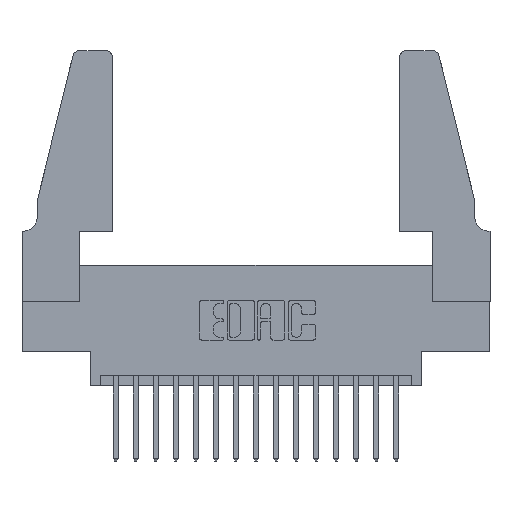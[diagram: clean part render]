
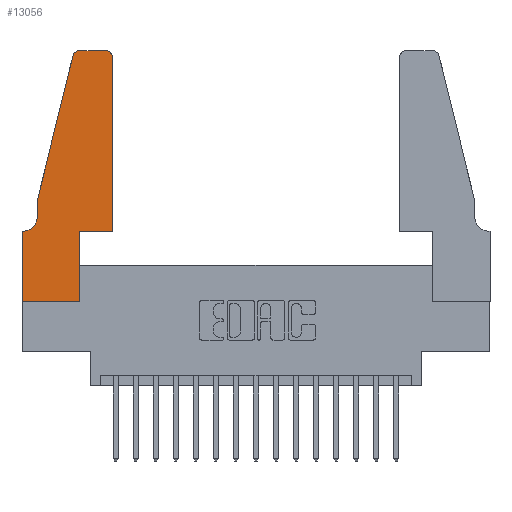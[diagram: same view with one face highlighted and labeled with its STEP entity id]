
A CAD part, top view. The second image highlights one B-rep face of the part: STEP entity #13056.
In plain terms, the highlighted planar face has unit normal (0, 0, 1).
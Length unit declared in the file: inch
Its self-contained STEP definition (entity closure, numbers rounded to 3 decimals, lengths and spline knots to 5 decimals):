
#598 = CARTESIAN_POINT ( 'NONE',  ( 0., 0., 0.37 ) ) ;
#627 = DIRECTION ( 'NONE',  ( -1., 0., 0. ) ) ;
#652 = DIRECTION ( 'NONE',  ( 0., 0., -1. ) ) ;
#676 = CARTESIAN_POINT ( 'NONE',  ( 0.0055, 0.42, 0.37 ) ) ;
#725 = VECTOR ( 'NONE', #9759, 39.37008 ) ;
#914 = VERTEX_POINT ( 'NONE', #3808 ) ;
#1017 = CARTESIAN_POINT ( 'NONE',  ( 0.2605, 1.25, 0.37 ) ) ;
#1130 = LINE ( 'NONE', #12833, #12560 ) ;
#1386 = ORIENTED_EDGE ( 'NONE', *, *, #15940, .T. ) ;
#1443 = EDGE_CURVE ( 'NONE', #9566, #13053, #5546, .T. ) ;
#1550 = ORIENTED_EDGE ( 'NONE', *, *, #2956, .T. ) ;
#1926 = ORIENTED_EDGE ( 'NONE', *, *, #15184, .T. ) ;
#1958 = VERTEX_POINT ( 'NONE', #2604 ) ;
#2333 = CARTESIAN_POINT ( 'NONE',  ( 0.0755, 0.42, 0.37 ) ) ;
#2424 = VERTEX_POINT ( 'NONE', #8724 ) ;
#2604 = CARTESIAN_POINT ( 'NONE',  ( 0.0755, 0.5, 0.37 ) ) ;
#2956 = EDGE_CURVE ( 'NONE', #2424, #6470, #9075, .T. ) ;
#3036 = CIRCLE ( 'NONE', #10200, 0.03 ) ;
#3119 = LINE ( 'NONE', #12220, #16553 ) ;
#3122 = ORIENTED_EDGE ( 'NONE', *, *, #3976, .T. ) ;
#3142 = VERTEX_POINT ( 'NONE', #12787 ) ;
#3474 = VECTOR ( 'NONE', #9433, 39.37008 ) ;
#3808 = CARTESIAN_POINT ( 'NONE',  ( 0.4505, 0.35, 0.37 ) ) ;
#3949 = DIRECTION ( 'NONE',  ( 0., 0., 1. ) ) ;
#3976 = EDGE_CURVE ( 'NONE', #6470, #1958, #3119, .T. ) ;
#4070 = EDGE_CURVE ( 'NONE', #13053, #6636, #8230, .T. ) ;
#4368 = CARTESIAN_POINT ( 'NONE',  ( 0.4505, 0.35, 0.37 ) ) ;
#4429 = DIRECTION ( 'NONE',  ( 1., 0., 0. ) ) ;
#4789 = DIRECTION ( 'NONE',  ( 0., 1., 0. ) ) ;
#5310 = CARTESIAN_POINT ( 'NONE',  ( 0., 0., 0.37 ) ) ;
#5424 = VECTOR ( 'NONE', #4429, 39.37008 ) ;
#5433 = VERTEX_POINT ( 'NONE', #15142 ) ;
#5546 = CIRCLE ( 'NONE', #17178, 0.07 ) ;
#5643 = CARTESIAN_POINT ( 'NONE',  ( 0.25487, 1.22718, 0.37 ) ) ;
#6321 = EDGE_LOOP ( 'NONE', ( #1926, #1550, #3122, #11526, #12856, #10383, #7652, #12730, #13578, #13949, #16267, #1386 ) ) ;
#6454 = AXIS2_PLACEMENT_3D ( 'NONE', #12992, #7694, #16978 ) ;
#6470 = VERTEX_POINT ( 'NONE', #5643 ) ;
#6636 = VERTEX_POINT ( 'NONE', #11262 ) ;
#6654 = VERTEX_POINT ( 'NONE', #12954 ) ;
#7019 = FACE_OUTER_BOUND ( 'NONE', #6321, .T. ) ;
#7129 = LINE ( 'NONE', #1017, #3474 ) ;
#7475 = CARTESIAN_POINT ( 'NONE',  ( 0.2865, 0.35, 0.37 ) ) ;
#7652 = ORIENTED_EDGE ( 'NONE', *, *, #8684, .T. ) ;
#7694 = DIRECTION ( 'NONE',  ( 0., 0., 1. ) ) ;
#8230 = LINE ( 'NONE', #8435, #725 ) ;
#8435 = CARTESIAN_POINT ( 'NONE',  ( 0.0755, 0.35, 0.37 ) ) ;
#8684 = EDGE_CURVE ( 'NONE', #6636, #15946, #16717, .T. ) ;
#8724 = CARTESIAN_POINT ( 'NONE',  ( 0.284, 1.25, 0.37 ) ) ;
#8913 = EDGE_CURVE ( 'NONE', #1958, #9566, #9431, .T. ) ;
#9008 = LINE ( 'NONE', #4368, #5424 ) ;
#9022 = DIRECTION ( 'NONE',  ( 1., 0., 0. ) ) ;
#9075 = CIRCLE ( 'NONE', #14974, 0.03 ) ;
#9431 = LINE ( 'NONE', #15269, #16083 ) ;
#9433 = DIRECTION ( 'NONE',  ( -1., 0., 0. ) ) ;
#9566 = VERTEX_POINT ( 'NONE', #2333 ) ;
#9670 = VERTEX_POINT ( 'NONE', #13445 ) ;
#9759 = DIRECTION ( 'NONE',  ( -1., 0., 0. ) ) ;
#10136 = DIRECTION ( 'NONE',  ( 0., 1., 0. ) ) ;
#10200 = AXIS2_PLACEMENT_3D ( 'NONE', #11999, #3949, #13340 ) ;
#10383 = ORIENTED_EDGE ( 'NONE', *, *, #4070, .T. ) ;
#11262 = CARTESIAN_POINT ( 'NONE',  ( 0., 0.35, 0.37 ) ) ;
#11313 = EDGE_CURVE ( 'NONE', #15946, #9670, #13748, .T. ) ;
#11526 = ORIENTED_EDGE ( 'NONE', *, *, #8913, .T. ) ;
#11999 = CARTESIAN_POINT ( 'NONE',  ( 0.4205, 1.22, 0.37 ) ) ;
#12220 = CARTESIAN_POINT ( 'NONE',  ( 0.0755, 0.5, 0.37 ) ) ;
#12560 = VECTOR ( 'NONE', #4789, 39.37008 ) ;
#12730 = ORIENTED_EDGE ( 'NONE', *, *, #11313, .T. ) ;
#12787 = CARTESIAN_POINT ( 'NONE',  ( 0.4205, 1.25, 0.37 ) ) ;
#12833 = CARTESIAN_POINT ( 'NONE',  ( 0.4505, 0.35, 0.37 ) ) ;
#12856 = ORIENTED_EDGE ( 'NONE', *, *, #1443, .T. ) ;
#12954 = CARTESIAN_POINT ( 'NONE',  ( 0.2865, 0.35, 0.37 ) ) ;
#12992 = CARTESIAN_POINT ( 'NONE',  ( 0., 0.35, 0.37 ) ) ;
#13053 = VERTEX_POINT ( 'NONE', #15553 ) ;
#13056 = ADVANCED_FACE ( 'NONE', ( #7019 ), #15659, .T. ) ;
#13340 = DIRECTION ( 'NONE',  ( 1., 0., 0. ) ) ;
#13358 = LINE ( 'NONE', #7475, #16699 ) ;
#13445 = CARTESIAN_POINT ( 'NONE',  ( 0.2865, 0., 0.37 ) ) ;
#13556 = DIRECTION ( 'NONE',  ( -0.239, -0.971, 0. ) ) ;
#13578 = ORIENTED_EDGE ( 'NONE', *, *, #15690, .T. ) ;
#13748 = LINE ( 'NONE', #598, #16852 ) ;
#13949 = ORIENTED_EDGE ( 'NONE', *, *, #14813, .T. ) ;
#14041 = DIRECTION ( 'NONE',  ( 1., 0., 0. ) ) ;
#14063 = DIRECTION ( 'NONE',  ( 0., 0., 1. ) ) ;
#14076 = CARTESIAN_POINT ( 'NONE',  ( 0.284, 1.22, 0.37 ) ) ;
#14794 = CARTESIAN_POINT ( 'NONE',  ( 0., 0., 0.37 ) ) ;
#14813 = EDGE_CURVE ( 'NONE', #6654, #914, #9008, .T. ) ;
#14859 = EDGE_CURVE ( 'NONE', #914, #5433, #1130, .T. ) ;
#14974 = AXIS2_PLACEMENT_3D ( 'NONE', #14076, #14063, #14041 ) ;
#15142 = CARTESIAN_POINT ( 'NONE',  ( 0.4505, 1.22, 0.37 ) ) ;
#15184 = EDGE_CURVE ( 'NONE', #3142, #2424, #7129, .T. ) ;
#15269 = CARTESIAN_POINT ( 'NONE',  ( 0.0755, 0.5, 0.37 ) ) ;
#15553 = CARTESIAN_POINT ( 'NONE',  ( 0.0055, 0.35, 0.37 ) ) ;
#15659 = PLANE ( 'NONE',  #6454 ) ;
#15690 = EDGE_CURVE ( 'NONE', #9670, #6654, #13358, .T. ) ;
#15940 = EDGE_CURVE ( 'NONE', #5433, #3142, #3036, .T. ) ;
#15946 = VERTEX_POINT ( 'NONE', #5310 ) ;
#16083 = VECTOR ( 'NONE', #16588, 39.37008 ) ;
#16134 = DIRECTION ( 'NONE',  ( 0., -1., 0. ) ) ;
#16267 = ORIENTED_EDGE ( 'NONE', *, *, #14859, .T. ) ;
#16292 = VECTOR ( 'NONE', #16134, 39.37008 ) ;
#16553 = VECTOR ( 'NONE', #13556, 39.37008 ) ;
#16588 = DIRECTION ( 'NONE',  ( 0., -1., 0. ) ) ;
#16699 = VECTOR ( 'NONE', #10136, 39.37008 ) ;
#16717 = LINE ( 'NONE', #14794, #16292 ) ;
#16852 = VECTOR ( 'NONE', #9022, 39.37008 ) ;
#16978 = DIRECTION ( 'NONE',  ( 1., 0., 0. ) ) ;
#17178 = AXIS2_PLACEMENT_3D ( 'NONE', #676, #652, #627 ) ;
